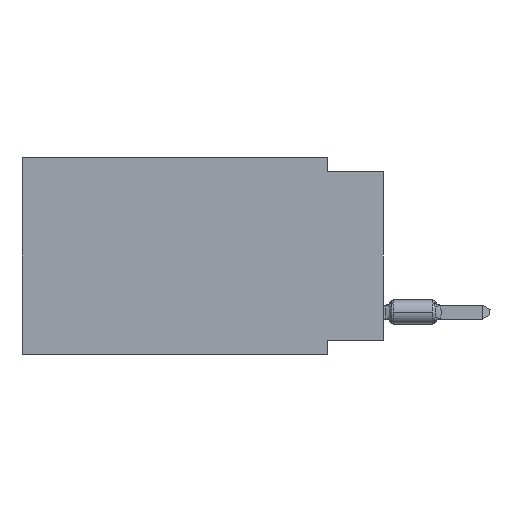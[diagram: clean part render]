
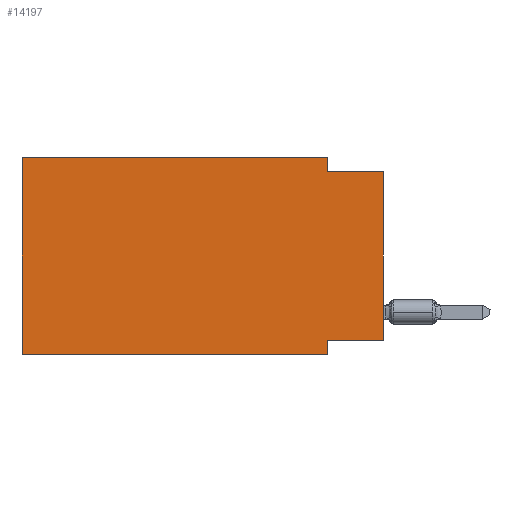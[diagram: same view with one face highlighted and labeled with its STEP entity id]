
A CAD part, left-side view. The second image highlights one B-rep face of the part: STEP entity #14197.
In plain terms, the highlighted planar face has unit normal (-1, 0, 0).
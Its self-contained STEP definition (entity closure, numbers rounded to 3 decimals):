
#32 = LINE ( 'NONE', #4268, #26312 ) ;
#443 = VERTEX_POINT ( 'NONE', #23237 ) ;
#4268 = CARTESIAN_POINT ( 'NONE',  ( 0., 16.383, -8.89 ) ) ;
#4499 = DIRECTION ( 'NONE',  ( 0., -1., 0. ) ) ;
#4964 = DIRECTION ( 'NONE',  ( 0., 0., -1. ) ) ;
#5744 = ORIENTED_EDGE ( 'NONE', *, *, #29608, .F. ) ;
#7190 = DIRECTION ( 'NONE',  ( 0., 0., 1. ) ) ;
#7369 = ORIENTED_EDGE ( 'NONE', *, *, #40045, .F. ) ;
#10042 = CARTESIAN_POINT ( 'NONE',  ( 0., 0., -8.255 ) ) ;
#12437 = ORIENTED_EDGE ( 'NONE', *, *, #57230, .F. ) ;
#12771 = DIRECTION ( 'NONE',  ( 0., 0., 1. ) ) ;
#12780 = DIRECTION ( 'NONE',  ( 0., -1., 0. ) ) ;
#13441 = EDGE_CURVE ( 'NONE', #47372, #26957, #46020, .T. ) ;
#13467 = DIRECTION ( 'NONE',  ( 0., 0., -1. ) ) ;
#14197 = ADVANCED_FACE ( 'NONE', ( #29653 ), #25124, .F. ) ;
#14658 = CARTESIAN_POINT ( 'NONE',  ( 0., 2.54, 0. ) ) ;
#15705 = DIRECTION ( 'NONE',  ( 0., 1., 0. ) ) ;
#17268 = ORIENTED_EDGE ( 'NONE', *, *, #27169, .T. ) ;
#19116 = VECTOR ( 'NONE', #12780, 1000. ) ;
#19661 = VECTOR ( 'NONE', #15705, 1000. ) ;
#21162 = EDGE_CURVE ( 'NONE', #48461, #23247, #58642, .T. ) ;
#23141 = CARTESIAN_POINT ( 'NONE',  ( 0., 2.54, -8.89 ) ) ;
#23237 = CARTESIAN_POINT ( 'NONE',  ( 0., 2.54, -8.89 ) ) ;
#23247 = VERTEX_POINT ( 'NONE', #32118 ) ;
#25124 = PLANE ( 'NONE',  #52621 ) ;
#25718 = DIRECTION ( 'NONE',  ( 0., 0., -1. ) ) ;
#26312 = VECTOR ( 'NONE', #32116, 1000. ) ;
#26957 = VERTEX_POINT ( 'NONE', #55054 ) ;
#27169 = EDGE_CURVE ( 'NONE', #47372, #443, #32, .T. ) ;
#27290 = CARTESIAN_POINT ( 'NONE',  ( 0., 0., -0.635 ) ) ;
#27402 = ORIENTED_EDGE ( 'NONE', *, *, #21162, .T. ) ;
#29608 = EDGE_CURVE ( 'NONE', #57235, #38631, #40700, .T. ) ;
#29653 = FACE_OUTER_BOUND ( 'NONE', #37232, .T. ) ;
#32116 = DIRECTION ( 'NONE',  ( 0., -1., 0. ) ) ;
#32118 = CARTESIAN_POINT ( 'NONE',  ( 0., 0., -0.635 ) ) ;
#33443 = VECTOR ( 'NONE', #13467, 1000. ) ;
#36882 = CARTESIAN_POINT ( 'NONE',  ( 0., 16.383, 0. ) ) ;
#37232 = EDGE_LOOP ( 'NONE', ( #27402, #51337, #5744, #7369, #55900, #17268, #12437, #50236 ) ) ;
#38631 = VERTEX_POINT ( 'NONE', #41238 ) ;
#40045 = EDGE_CURVE ( 'NONE', #26957, #57235, #51409, .T. ) ;
#40700 = LINE ( 'NONE', #40987, #33443 ) ;
#40987 = CARTESIAN_POINT ( 'NONE',  ( 0., 2.54, 0. ) ) ;
#41238 = CARTESIAN_POINT ( 'NONE',  ( 0., 2.54, -0.635 ) ) ;
#41508 = EDGE_CURVE ( 'NONE', #48461, #57734, #56329, .T. ) ;
#41879 = LINE ( 'NONE', #23141, #58309 ) ;
#44210 = CARTESIAN_POINT ( 'NONE',  ( 0., 16.383, -8.89 ) ) ;
#45431 = CARTESIAN_POINT ( 'NONE',  ( 0., 16.383, 0. ) ) ;
#46020 = LINE ( 'NONE', #45431, #49662 ) ;
#46127 = CARTESIAN_POINT ( 'NONE',  ( 0., 0., -8.255 ) ) ;
#47372 = VERTEX_POINT ( 'NONE', #44210 ) ;
#48412 = CARTESIAN_POINT ( 'NONE',  ( 0., 16.383, 0. ) ) ;
#48461 = VERTEX_POINT ( 'NONE', #46127 ) ;
#48949 = CARTESIAN_POINT ( 'NONE',  ( 0., 0., 0. ) ) ;
#49662 = VECTOR ( 'NONE', #12771, 1000. ) ;
#49683 = LINE ( 'NONE', #27290, #19116 ) ;
#50236 = ORIENTED_EDGE ( 'NONE', *, *, #41508, .F. ) ;
#51337 = ORIENTED_EDGE ( 'NONE', *, *, #59498, .F. ) ;
#51409 = LINE ( 'NONE', #36882, #57236 ) ;
#52091 = CARTESIAN_POINT ( 'NONE',  ( 0., 2.54, -8.255 ) ) ;
#52621 = AXIS2_PLACEMENT_3D ( 'NONE', #48412, #53247, #25718 ) ;
#53247 = DIRECTION ( 'NONE',  ( 1., 0., 0. ) ) ;
#55054 = CARTESIAN_POINT ( 'NONE',  ( 0., 16.383, 0. ) ) ;
#55900 = ORIENTED_EDGE ( 'NONE', *, *, #13441, .F. ) ;
#56329 = LINE ( 'NONE', #10042, #19661 ) ;
#57230 = EDGE_CURVE ( 'NONE', #57734, #443, #41879, .T. ) ;
#57235 = VERTEX_POINT ( 'NONE', #14658 ) ;
#57236 = VECTOR ( 'NONE', #4499, 1000. ) ;
#57734 = VERTEX_POINT ( 'NONE', #52091 ) ;
#58309 = VECTOR ( 'NONE', #4964, 1000. ) ;
#58642 = LINE ( 'NONE', #48949, #59653 ) ;
#59498 = EDGE_CURVE ( 'NONE', #38631, #23247, #49683, .T. ) ;
#59653 = VECTOR ( 'NONE', #7190, 1000. ) ;
